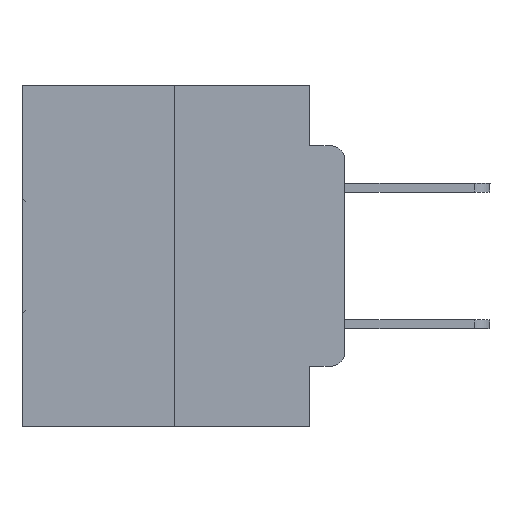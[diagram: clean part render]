
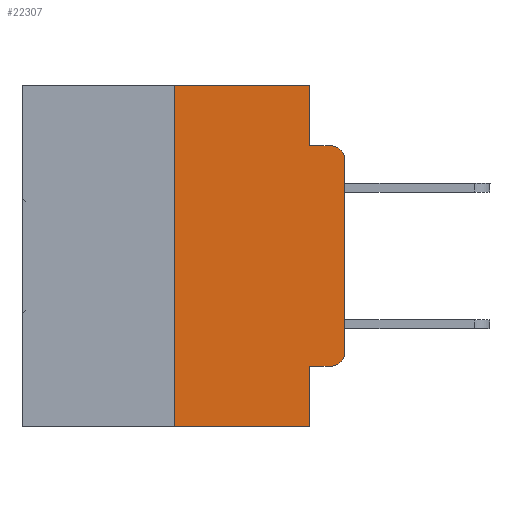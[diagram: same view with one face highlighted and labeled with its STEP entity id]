
A CAD part, left-side view. The second image highlights one B-rep face of the part: STEP entity #22307.
In plain terms, the highlighted planar face has unit normal (-1, 0, 0).
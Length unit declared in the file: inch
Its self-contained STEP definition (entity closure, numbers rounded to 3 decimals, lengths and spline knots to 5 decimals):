
#759 = VECTOR ( 'NONE', #7718, 39.37008 ) ;
#1528 = VECTOR ( 'NONE', #23663, 39.37008 ) ;
#2311 = CIRCLE ( 'NONE', #7812, 0.02 ) ;
#2639 = CARTESIAN_POINT ( 'NONE',  ( 0., 0., -0.3915 ) ) ;
#3018 = DIRECTION ( 'NONE',  ( 0., -1., 0. ) ) ;
#3593 = EDGE_CURVE ( 'NONE', #7893, #21191, #6487, .T. ) ;
#3722 = CARTESIAN_POINT ( 'NONE',  ( 0., 0.02, -0.3915 ) ) ;
#4449 = VERTEX_POINT ( 'NONE', #28324 ) ;
#4516 = CARTESIAN_POINT ( 'NONE',  ( 0., 0.25, 0. ) ) ;
#4651 = DIRECTION ( 'NONE',  ( -1., 0., 0. ) ) ;
#4688 = DIRECTION ( 'NONE',  ( 0., 0., -1. ) ) ;
#4958 = LINE ( 'NONE', #21570, #24661 ) ;
#5313 = EDGE_CURVE ( 'NONE', #20218, #7893, #20713, .T. ) ;
#5391 = CARTESIAN_POINT ( 'NONE',  ( 0., 0.051, -0.5 ) ) ;
#5822 = LINE ( 'NONE', #15300, #31047 ) ;
#6320 = DIRECTION ( 'NONE',  ( 0., 0., -1. ) ) ;
#6487 = CIRCLE ( 'NONE', #24649, 0.02 ) ;
#6653 = AXIS2_PLACEMENT_3D ( 'NONE', #11469, #28385, #13932 ) ;
#7426 = ORIENTED_EDGE ( 'NONE', *, *, #20882, .F. ) ;
#7718 = DIRECTION ( 'NONE',  ( 0., 0., 1. ) ) ;
#7812 = AXIS2_PLACEMENT_3D ( 'NONE', #3722, #21113, #6320 ) ;
#7893 = VERTEX_POINT ( 'NONE', #29844 ) ;
#9922 = CARTESIAN_POINT ( 'NONE',  ( 0., 0.25, 0. ) ) ;
#10213 = ORIENTED_EDGE ( 'NONE', *, *, #28914, .F. ) ;
#10468 = DIRECTION ( 'NONE',  ( 0., 0., -1. ) ) ;
#10655 = ORIENTED_EDGE ( 'NONE', *, *, #17626, .T. ) ;
#10693 = VERTEX_POINT ( 'NONE', #13416 ) ;
#10973 = VECTOR ( 'NONE', #19432, 39.37008 ) ;
#11469 = CARTESIAN_POINT ( 'NONE',  ( 0., 0.473, 0. ) ) ;
#13322 = EDGE_CURVE ( 'NONE', #14779, #29967, #4958, .T. ) ;
#13416 = CARTESIAN_POINT ( 'NONE',  ( 0., 0.02, -0.4115 ) ) ;
#13871 = EDGE_LOOP ( 'NONE', ( #23838, #20879, #22414, #10213, #18243, #29150, #22448, #7426, #21310, #10655 ) ) ;
#13932 = DIRECTION ( 'NONE',  ( 0., 0., -1. ) ) ;
#14779 = VERTEX_POINT ( 'NONE', #9922 ) ;
#14988 = LINE ( 'NONE', #23772, #1528 ) ;
#15300 = CARTESIAN_POINT ( 'NONE',  ( 0., 0.051, 0. ) ) ;
#17583 = CARTESIAN_POINT ( 'NONE',  ( 0., 0.051, -0.4115 ) ) ;
#17626 = EDGE_CURVE ( 'NONE', #10693, #20218, #2311, .T. ) ;
#17876 = CARTESIAN_POINT ( 'NONE',  ( 0., 0.051, 0. ) ) ;
#17892 = LINE ( 'NONE', #18061, #24327 ) ;
#18061 = CARTESIAN_POINT ( 'NONE',  ( 0., 0.051, -0.0885 ) ) ;
#18243 = ORIENTED_EDGE ( 'NONE', *, *, #13322, .F. ) ;
#18713 = PLANE ( 'NONE',  #6653 ) ;
#18749 = LINE ( 'NONE', #19849, #25921 ) ;
#19034 = CARTESIAN_POINT ( 'NONE',  ( 0., 0.02, -0.1085 ) ) ;
#19064 = CARTESIAN_POINT ( 'NONE',  ( 0., 0.25, -0.5 ) ) ;
#19263 = EDGE_CURVE ( 'NONE', #19880, #10693, #18749, .T. ) ;
#19432 = DIRECTION ( 'NONE',  ( 0., 0., 1. ) ) ;
#19849 = CARTESIAN_POINT ( 'NONE',  ( 0., 0.051, -0.4115 ) ) ;
#19880 = VERTEX_POINT ( 'NONE', #17583 ) ;
#20218 = VERTEX_POINT ( 'NONE', #2639 ) ;
#20713 = LINE ( 'NONE', #24771, #759 ) ;
#20879 = ORIENTED_EDGE ( 'NONE', *, *, #3593, .T. ) ;
#20882 = EDGE_CURVE ( 'NONE', #19880, #31050, #5822, .T. ) ;
#21113 = DIRECTION ( 'NONE',  ( -1., 0., 0. ) ) ;
#21191 = VERTEX_POINT ( 'NONE', #21313 ) ;
#21310 = ORIENTED_EDGE ( 'NONE', *, *, #19263, .T. ) ;
#21313 = CARTESIAN_POINT ( 'NONE',  ( 0., 0.02, -0.0885 ) ) ;
#21570 = CARTESIAN_POINT ( 'NONE',  ( 0., 0.473, 0. ) ) ;
#22010 = FACE_OUTER_BOUND ( 'NONE', #13871, .T. ) ;
#22307 = ADVANCED_FACE ( 'NONE', ( #22010 ), #18713, .F. ) ;
#22414 = ORIENTED_EDGE ( 'NONE', *, *, #30533, .F. ) ;
#22448 = ORIENTED_EDGE ( 'NONE', *, *, #27741, .T. ) ;
#22519 = EDGE_CURVE ( 'NONE', #26137, #14779, #23893, .T. ) ;
#22838 = DIRECTION ( 'NONE',  ( 0., -1., 0. ) ) ;
#23663 = DIRECTION ( 'NONE',  ( 0., 0., -1. ) ) ;
#23772 = CARTESIAN_POINT ( 'NONE',  ( 0., 0.051, 0. ) ) ;
#23838 = ORIENTED_EDGE ( 'NONE', *, *, #5313, .T. ) ;
#23893 = LINE ( 'NONE', #4516, #10973 ) ;
#24327 = VECTOR ( 'NONE', #22838, 39.37008 ) ;
#24649 = AXIS2_PLACEMENT_3D ( 'NONE', #19034, #4651, #4688 ) ;
#24661 = VECTOR ( 'NONE', #31097, 39.37008 ) ;
#24771 = CARTESIAN_POINT ( 'NONE',  ( 0., 0., 0. ) ) ;
#25921 = VECTOR ( 'NONE', #27031, 39.37008 ) ;
#26137 = VERTEX_POINT ( 'NONE', #19064 ) ;
#27031 = DIRECTION ( 'NONE',  ( 0., -1., 0. ) ) ;
#27196 = VECTOR ( 'NONE', #3018, 39.37008 ) ;
#27598 = CARTESIAN_POINT ( 'NONE',  ( 0., 0.473, -0.5 ) ) ;
#27741 = EDGE_CURVE ( 'NONE', #26137, #31050, #27926, .T. ) ;
#27926 = LINE ( 'NONE', #27598, #27196 ) ;
#28324 = CARTESIAN_POINT ( 'NONE',  ( 0., 0.051, -0.0885 ) ) ;
#28385 = DIRECTION ( 'NONE',  ( 1., 0., 0. ) ) ;
#28914 = EDGE_CURVE ( 'NONE', #29967, #4449, #14988, .T. ) ;
#29150 = ORIENTED_EDGE ( 'NONE', *, *, #22519, .F. ) ;
#29844 = CARTESIAN_POINT ( 'NONE',  ( 0., 0., -0.1085 ) ) ;
#29967 = VERTEX_POINT ( 'NONE', #17876 ) ;
#30533 = EDGE_CURVE ( 'NONE', #4449, #21191, #17892, .T. ) ;
#31047 = VECTOR ( 'NONE', #10468, 39.37008 ) ;
#31050 = VERTEX_POINT ( 'NONE', #5391 ) ;
#31097 = DIRECTION ( 'NONE',  ( 0., -1., 0. ) ) ;
